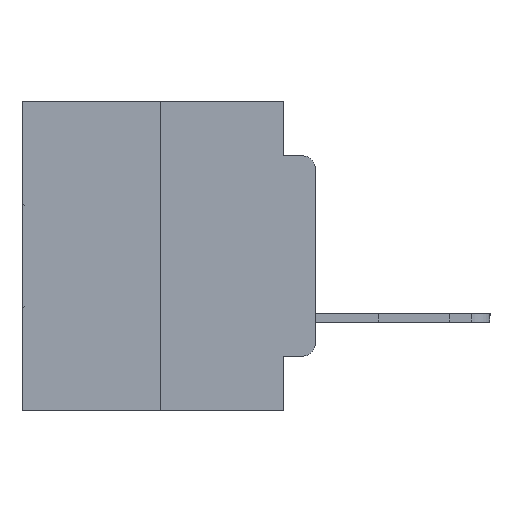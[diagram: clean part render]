
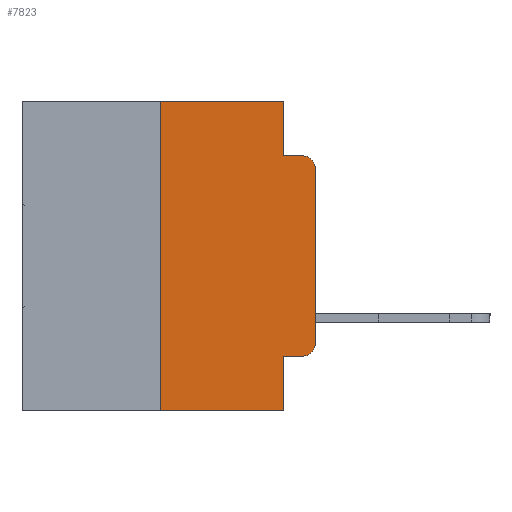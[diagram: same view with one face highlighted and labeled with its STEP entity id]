
A CAD part, left-side view. The second image highlights one B-rep face of the part: STEP entity #7823.
In plain terms, the highlighted planar face has unit normal (-1, 0, 0).
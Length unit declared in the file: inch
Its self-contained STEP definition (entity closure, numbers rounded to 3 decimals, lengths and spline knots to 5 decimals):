
#132 = DIRECTION ( 'NONE',  ( 0., -1., 0. ) ) ;
#1109 = ORIENTED_EDGE ( 'NONE', *, *, #26369, .F. ) ;
#2406 = CARTESIAN_POINT ( 'NONE',  ( 0., 0.473, 0. ) ) ;
#2731 = VERTEX_POINT ( 'NONE', #25439 ) ;
#2772 = EDGE_CURVE ( 'NONE', #16075, #12234, #14525, .T. ) ;
#2774 = EDGE_CURVE ( 'NONE', #12234, #22032, #25628, .T. ) ;
#2852 = EDGE_CURVE ( 'NONE', #10801, #22032, #4830, .T. ) ;
#2854 = EDGE_CURVE ( 'NONE', #14307, #10801, #11008, .T. ) ;
#2859 = EDGE_CURVE ( 'NONE', #12881, #2731, #5619, .T. ) ;
#3298 = EDGE_CURVE ( 'NONE', #8144, #14133, #24029, .T. ) ;
#3303 = EDGE_CURVE ( 'NONE', #8144, #15065, #14125, .T. ) ;
#3307 = EDGE_CURVE ( 'NONE', #15065, #16075, #17884, .T. ) ;
#4070 = VECTOR ( 'NONE', #26045, 39.37008 ) ;
#4190 = CARTESIAN_POINT ( 'NONE',  ( 0., 0.051, 0. ) ) ;
#4443 = ORIENTED_EDGE ( 'NONE', *, *, #2772, .T. ) ;
#4515 = CARTESIAN_POINT ( 'NONE',  ( 0., 0., -0.1085 ) ) ;
#4830 = LINE ( 'NONE', #17786, #27806 ) ;
#5227 = ORIENTED_EDGE ( 'NONE', *, *, #2774, .T. ) ;
#5619 = LINE ( 'NONE', #19931, #4070 ) ;
#6374 = ORIENTED_EDGE ( 'NONE', *, *, #3307, .T. ) ;
#6539 = DIRECTION ( 'NONE',  ( 0., -1., 0. ) ) ;
#7209 = PLANE ( 'NONE',  #10411 ) ;
#7698 = CARTESIAN_POINT ( 'NONE',  ( 0., 0.02, -0.4115 ) ) ;
#7823 = ADVANCED_FACE ( 'NONE', ( #14995 ), #7209, .F. ) ;
#8144 = VERTEX_POINT ( 'NONE', #21694 ) ;
#8810 = EDGE_CURVE ( 'NONE', #12881, #14133, #16013, .T. ) ;
#8928 = DIRECTION ( 'NONE',  ( 0., 0., -1. ) ) ;
#9519 = CARTESIAN_POINT ( 'NONE',  ( 0., 0.051, 0. ) ) ;
#9535 = DIRECTION ( 'NONE',  ( 1., 0., 0. ) ) ;
#9619 = DIRECTION ( 'NONE',  ( -1., 0., 0. ) ) ;
#10123 = CARTESIAN_POINT ( 'NONE',  ( 0., 0.051, -0.0885 ) ) ;
#10393 = CARTESIAN_POINT ( 'NONE',  ( 0., 0.473, 0. ) ) ;
#10411 = AXIS2_PLACEMENT_3D ( 'NONE', #2406, #9535, #24558 ) ;
#10801 = VERTEX_POINT ( 'NONE', #10123 ) ;
#10835 = CARTESIAN_POINT ( 'NONE',  ( 0., 0.02, -0.1085 ) ) ;
#11008 = LINE ( 'NONE', #4190, #16248 ) ;
#11700 = ORIENTED_EDGE ( 'NONE', *, *, #3298, .F. ) ;
#12234 = VERTEX_POINT ( 'NONE', #4515 ) ;
#12881 = VERTEX_POINT ( 'NONE', #14228 ) ;
#12946 = CARTESIAN_POINT ( 'NONE',  ( 0., 0., 0. ) ) ;
#13040 = DIRECTION ( 'NONE',  ( 0., 0., -1. ) ) ;
#14008 = DIRECTION ( 'NONE',  ( 0., 0., -1. ) ) ;
#14125 = LINE ( 'NONE', #26524, #18576 ) ;
#14133 = VERTEX_POINT ( 'NONE', #23097 ) ;
#14228 = CARTESIAN_POINT ( 'NONE',  ( 0., 0.25, -0.5 ) ) ;
#14307 = VERTEX_POINT ( 'NONE', #19791 ) ;
#14525 = LINE ( 'NONE', #12946, #25022 ) ;
#14995 = FACE_OUTER_BOUND ( 'NONE', #17970, .T. ) ;
#15065 = VERTEX_POINT ( 'NONE', #7698 ) ;
#16013 = LINE ( 'NONE', #28363, #26355 ) ;
#16075 = VERTEX_POINT ( 'NONE', #25993 ) ;
#16136 = DIRECTION ( 'NONE',  ( 0., -1., 0. ) ) ;
#16248 = VECTOR ( 'NONE', #8928, 39.37008 ) ;
#16267 = ORIENTED_EDGE ( 'NONE', *, *, #8810, .T. ) ;
#16797 = CARTESIAN_POINT ( 'NONE',  ( 0., 0.02, -0.0885 ) ) ;
#17256 = ORIENTED_EDGE ( 'NONE', *, *, #2852, .F. ) ;
#17431 = DIRECTION ( 'NONE',  ( 0., 0., 1. ) ) ;
#17786 = CARTESIAN_POINT ( 'NONE',  ( 0., 0.051, -0.0885 ) ) ;
#17884 = CIRCLE ( 'NONE', #22370, 0.02 ) ;
#17970 = EDGE_LOOP ( 'NONE', ( #4443, #5227, #17256, #24070, #1109, #24710, #16267, #11700, #23138, #6374 ) ) ;
#18576 = VECTOR ( 'NONE', #132, 39.37008 ) ;
#19791 = CARTESIAN_POINT ( 'NONE',  ( 0., 0.051, 0. ) ) ;
#19931 = CARTESIAN_POINT ( 'NONE',  ( 0., 0.25, 0. ) ) ;
#21694 = CARTESIAN_POINT ( 'NONE',  ( 0., 0.051, -0.4115 ) ) ;
#22032 = VERTEX_POINT ( 'NONE', #16797 ) ;
#22370 = AXIS2_PLACEMENT_3D ( 'NONE', #22589, #9619, #24623 ) ;
#22589 = CARTESIAN_POINT ( 'NONE',  ( 0., 0.02, -0.3915 ) ) ;
#23097 = CARTESIAN_POINT ( 'NONE',  ( 0., 0.051, -0.5 ) ) ;
#23138 = ORIENTED_EDGE ( 'NONE', *, *, #3303, .T. ) ;
#23403 = VECTOR ( 'NONE', #14008, 39.37008 ) ;
#24029 = LINE ( 'NONE', #9519, #23403 ) ;
#24070 = ORIENTED_EDGE ( 'NONE', *, *, #2854, .F. ) ;
#24558 = DIRECTION ( 'NONE',  ( 0., 0., -1. ) ) ;
#24623 = DIRECTION ( 'NONE',  ( 0., 0., -1. ) ) ;
#24710 = ORIENTED_EDGE ( 'NONE', *, *, #2859, .F. ) ;
#25022 = VECTOR ( 'NONE', #17431, 39.37008 ) ;
#25221 = AXIS2_PLACEMENT_3D ( 'NONE', #10835, #25689, #13040 ) ;
#25439 = CARTESIAN_POINT ( 'NONE',  ( 0., 0.25, 0. ) ) ;
#25628 = CIRCLE ( 'NONE', #25221, 0.02 ) ;
#25689 = DIRECTION ( 'NONE',  ( -1., 0., 0. ) ) ;
#25993 = CARTESIAN_POINT ( 'NONE',  ( 0., 0., -0.3915 ) ) ;
#26045 = DIRECTION ( 'NONE',  ( 0., 0., 1. ) ) ;
#26355 = VECTOR ( 'NONE', #16136, 39.37008 ) ;
#26369 = EDGE_CURVE ( 'NONE', #2731, #14307, #27602, .T. ) ;
#26524 = CARTESIAN_POINT ( 'NONE',  ( 0., 0.051, -0.4115 ) ) ;
#26991 = VECTOR ( 'NONE', #27212, 39.37008 ) ;
#27212 = DIRECTION ( 'NONE',  ( 0., -1., 0. ) ) ;
#27602 = LINE ( 'NONE', #10393, #26991 ) ;
#27806 = VECTOR ( 'NONE', #6539, 39.37008 ) ;
#28363 = CARTESIAN_POINT ( 'NONE',  ( 0., 0.473, -0.5 ) ) ;
